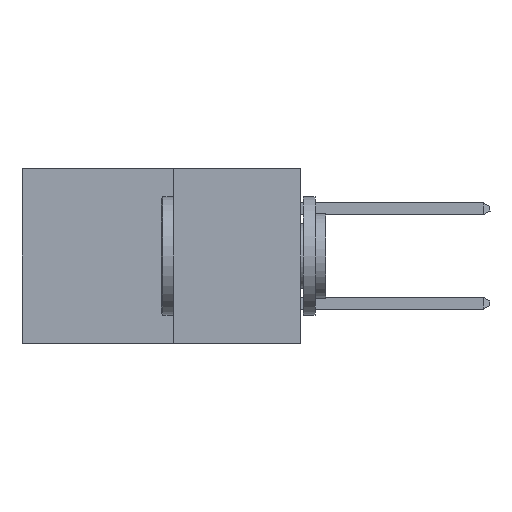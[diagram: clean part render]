
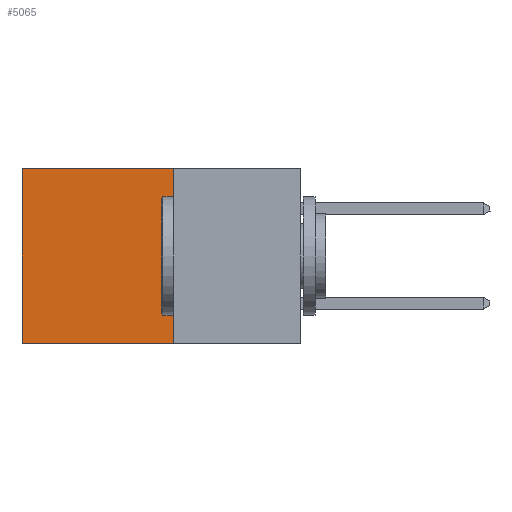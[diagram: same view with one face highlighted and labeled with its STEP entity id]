
A CAD part, left-side view. The second image highlights one B-rep face of the part: STEP entity #5065.
In plain terms, the highlighted planar face has unit normal (-1, 0, 0).
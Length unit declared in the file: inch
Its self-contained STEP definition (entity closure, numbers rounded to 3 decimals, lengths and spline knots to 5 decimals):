
#32 = EDGE_CURVE ( 'NONE', #14458, #11974, #15414, .T. ) ;
#461 = CARTESIAN_POINT ( 'NONE',  ( 0.277, 0.27, -0.37 ) ) ;
#541 = VECTOR ( 'NONE', #13596, 39.37008 ) ;
#1263 = CARTESIAN_POINT ( 'NONE',  ( 0.277, 0.27, 0. ) ) ;
#1319 = EDGE_CURVE ( 'NONE', #12507, #10650, #6936, .T. ) ;
#1591 = VECTOR ( 'NONE', #6904, 39.37008 ) ;
#1595 = CARTESIAN_POINT ( 'NONE',  ( 0.277, 0.59, -0.37 ) ) ;
#2129 = DIRECTION ( 'NONE',  ( 0., 0., -1. ) ) ;
#2878 = LINE ( 'NONE', #5128, #17037 ) ;
#3711 = ORIENTED_EDGE ( 'NONE', *, *, #1319, .T. ) ;
#5065 = ADVANCED_FACE ( 'NONE', ( #15930 ), #16552, .F. ) ;
#5128 = CARTESIAN_POINT ( 'NONE',  ( 0.277, 0.27, -0.37 ) ) ;
#5482 = AXIS2_PLACEMENT_3D ( 'NONE', #16471, #16429, #16426 ) ;
#5832 = ORIENTED_EDGE ( 'NONE', *, *, #32, .F. ) ;
#6149 = CARTESIAN_POINT ( 'NONE',  ( 0.277, 0.27, 0. ) ) ;
#6761 = EDGE_LOOP ( 'NONE', ( #16943, #5832, #14979, #3711 ) ) ;
#6904 = DIRECTION ( 'NONE',  ( 0., 1., 0. ) ) ;
#6936 = LINE ( 'NONE', #6149, #1591 ) ;
#8043 = EDGE_CURVE ( 'NONE', #10650, #11974, #8401, .T. ) ;
#8401 = LINE ( 'NONE', #13802, #541 ) ;
#9648 = DIRECTION ( 'NONE',  ( 0., 1., 0. ) ) ;
#10375 = CARTESIAN_POINT ( 'NONE',  ( 0.277, 0.59, 0. ) ) ;
#10650 = VERTEX_POINT ( 'NONE', #10375 ) ;
#11590 = VECTOR ( 'NONE', #9648, 39.37008 ) ;
#11974 = VERTEX_POINT ( 'NONE', #1595 ) ;
#12507 = VERTEX_POINT ( 'NONE', #1263 ) ;
#13596 = DIRECTION ( 'NONE',  ( 0., 0., -1. ) ) ;
#13683 = EDGE_CURVE ( 'NONE', #12507, #14458, #2878, .T. ) ;
#13802 = CARTESIAN_POINT ( 'NONE',  ( 0.277, 0.59, -0.37 ) ) ;
#14458 = VERTEX_POINT ( 'NONE', #15628 ) ;
#14979 = ORIENTED_EDGE ( 'NONE', *, *, #13683, .F. ) ;
#15414 = LINE ( 'NONE', #461, #11590 ) ;
#15628 = CARTESIAN_POINT ( 'NONE',  ( 0.277, 0.27, -0.37 ) ) ;
#15930 = FACE_OUTER_BOUND ( 'NONE', #6761, .T. ) ;
#16426 = DIRECTION ( 'NONE',  ( 0., 0., -1. ) ) ;
#16429 = DIRECTION ( 'NONE',  ( 1., 0., 0. ) ) ;
#16471 = CARTESIAN_POINT ( 'NONE',  ( 0.277, 0.27, -0.37 ) ) ;
#16552 = PLANE ( 'NONE',  #5482 ) ;
#16943 = ORIENTED_EDGE ( 'NONE', *, *, #8043, .T. ) ;
#17037 = VECTOR ( 'NONE', #2129, 39.37008 ) ;
